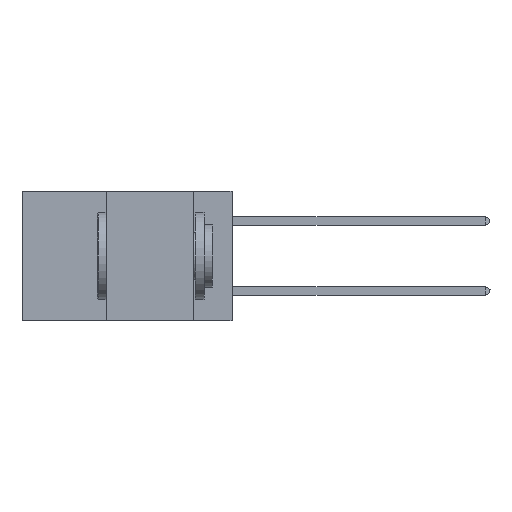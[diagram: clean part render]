
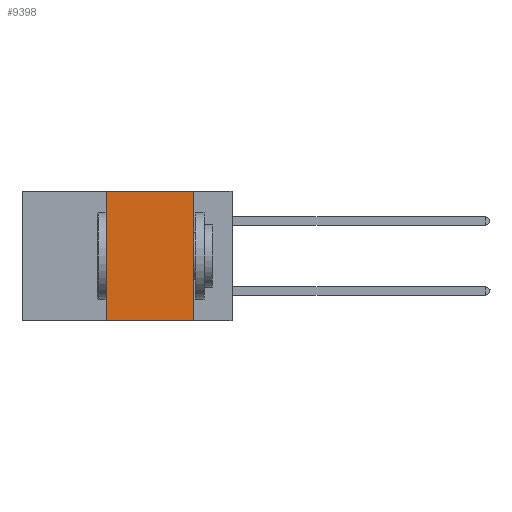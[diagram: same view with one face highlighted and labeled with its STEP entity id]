
A CAD part, left-side view. The second image highlights one B-rep face of the part: STEP entity #9398.
In plain terms, the highlighted planar face has unit normal (-1, 0, 0).
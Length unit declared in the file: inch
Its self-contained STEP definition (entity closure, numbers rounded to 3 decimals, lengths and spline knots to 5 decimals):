
#675 = CARTESIAN_POINT ( 'NONE',  ( 0., 0.6, -0.37 ) ) ;
#830 = FACE_OUTER_BOUND ( 'NONE', #19133, .T. ) ;
#1145 = CARTESIAN_POINT ( 'NONE',  ( 0., 0.6, 0. ) ) ;
#1536 = LINE ( 'NONE', #675, #12016 ) ;
#1725 = CARTESIAN_POINT ( 'NONE',  ( 0., 0.11, 0. ) ) ;
#2344 = VERTEX_POINT ( 'NONE', #17040 ) ;
#3120 = VECTOR ( 'NONE', #21552, 39.37008 ) ;
#3851 = ORIENTED_EDGE ( 'NONE', *, *, #9079, .F. ) ;
#3981 = PLANE ( 'NONE',  #4346 ) ;
#4346 = AXIS2_PLACEMENT_3D ( 'NONE', #11281, #12858, #21934 ) ;
#4582 = EDGE_CURVE ( 'NONE', #2344, #9129, #15924, .T. ) ;
#5562 = CARTESIAN_POINT ( 'NONE',  ( 0., 0.11, 0. ) ) ;
#6062 = DIRECTION ( 'NONE',  ( 0., -1., 0. ) ) ;
#6349 = DIRECTION ( 'NONE',  ( 0., 0., -1. ) ) ;
#6684 = DIRECTION ( 'NONE',  ( 0., -1., 0. ) ) ;
#7967 = LINE ( 'NONE', #8945, #3120 ) ;
#8789 = ORIENTED_EDGE ( 'NONE', *, *, #4582, .F. ) ;
#8945 = CARTESIAN_POINT ( 'NONE',  ( 0., 0.36, 0. ) ) ;
#9079 = EDGE_CURVE ( 'NONE', #14206, #2344, #7967, .T. ) ;
#9129 = VERTEX_POINT ( 'NONE', #5562 ) ;
#9398 = ADVANCED_FACE ( 'NONE', ( #830 ), #3981, .F. ) ;
#11281 = CARTESIAN_POINT ( 'NONE',  ( 0., 0.6, 0. ) ) ;
#12016 = VECTOR ( 'NONE', #6062, 39.37008 ) ;
#12167 = ORIENTED_EDGE ( 'NONE', *, *, #16974, .T. ) ;
#12431 = CARTESIAN_POINT ( 'NONE',  ( 0., 0.36, -0.37 ) ) ;
#12760 = ORIENTED_EDGE ( 'NONE', *, *, #16618, .F. ) ;
#12858 = DIRECTION ( 'NONE',  ( 1., 0., 0. ) ) ;
#13389 = VECTOR ( 'NONE', #6684, 39.37008 ) ;
#14206 = VERTEX_POINT ( 'NONE', #12431 ) ;
#15924 = LINE ( 'NONE', #1145, #13389 ) ;
#16618 = EDGE_CURVE ( 'NONE', #9129, #22790, #17067, .T. ) ;
#16974 = EDGE_CURVE ( 'NONE', #14206, #22790, #1536, .T. ) ;
#17040 = CARTESIAN_POINT ( 'NONE',  ( 0., 0.36, 0. ) ) ;
#17067 = LINE ( 'NONE', #1725, #18186 ) ;
#18186 = VECTOR ( 'NONE', #6349, 39.37008 ) ;
#18976 = CARTESIAN_POINT ( 'NONE',  ( 0., 0.11, -0.37 ) ) ;
#19133 = EDGE_LOOP ( 'NONE', ( #12760, #8789, #3851, #12167 ) ) ;
#21552 = DIRECTION ( 'NONE',  ( 0., 0., 1. ) ) ;
#21934 = DIRECTION ( 'NONE',  ( 0., 0., -1. ) ) ;
#22790 = VERTEX_POINT ( 'NONE', #18976 ) ;
